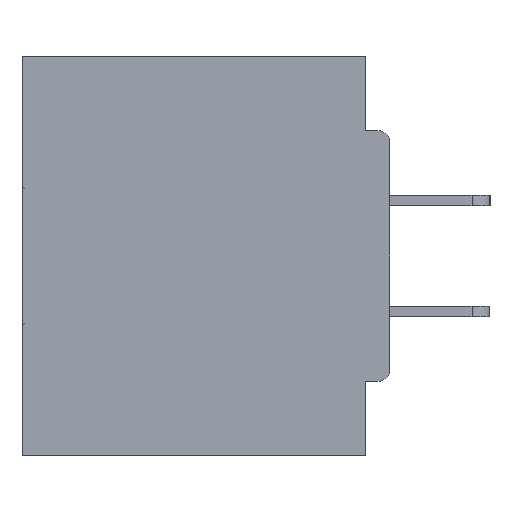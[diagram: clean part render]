
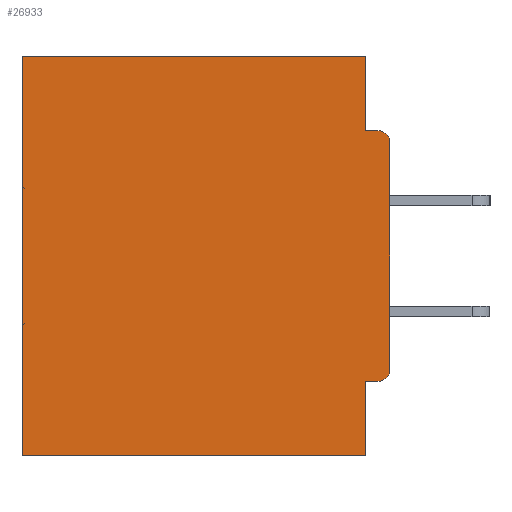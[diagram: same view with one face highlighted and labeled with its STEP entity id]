
A CAD part, left-side view. The second image highlights one B-rep face of the part: STEP entity #26933.
In plain terms, the highlighted planar face has unit normal (-1, 0, 0).
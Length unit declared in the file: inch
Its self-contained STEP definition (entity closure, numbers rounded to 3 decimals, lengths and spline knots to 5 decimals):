
#36 = FACE_OUTER_BOUND ( 'NONE', #34327, .T. ) ;
#632 = VERTEX_POINT ( 'NONE', #25162 ) ;
#668 = ORIENTED_EDGE ( 'NONE', *, *, #20912, .F. ) ;
#851 = ORIENTED_EDGE ( 'NONE', *, *, #15836, .T. ) ;
#2122 = DIRECTION ( 'NONE',  ( 0., 0., -1. ) ) ;
#2670 = LINE ( 'NONE', #19933, #12013 ) ;
#3550 = EDGE_CURVE ( 'NONE', #24531, #37569, #21996, .T. ) ;
#3868 = VERTEX_POINT ( 'NONE', #36581 ) ;
#4041 = CARTESIAN_POINT ( 'NONE',  ( 0.298, 0., 0. ) ) ;
#4188 = ORIENTED_EDGE ( 'NONE', *, *, #13792, .F. ) ;
#4927 = VERTEX_POINT ( 'NONE', #39853 ) ;
#5323 = AXIS2_PLACEMENT_3D ( 'NONE', #31454, #15018, #11538 ) ;
#5377 = CARTESIAN_POINT ( 'NONE',  ( 0.298, 0.015, -0.0935 ) ) ;
#5729 = CIRCLE ( 'NONE', #24705, 0.015 ) ;
#6074 = CARTESIAN_POINT ( 'NONE',  ( 0.298, 0., -0.1085 ) ) ;
#8146 = CARTESIAN_POINT ( 'NONE',  ( 0.298, 0., -0.0935 ) ) ;
#9762 = EDGE_CURVE ( 'NONE', #40306, #33398, #24197, .T. ) ;
#9853 = CARTESIAN_POINT ( 'NONE',  ( 0.298, 0.015, -0.3915 ) ) ;
#10743 = ORIENTED_EDGE ( 'NONE', *, *, #31924, .F. ) ;
#11538 = DIRECTION ( 'NONE',  ( 0., 0., -1. ) ) ;
#11604 = LINE ( 'NONE', #4041, #32440 ) ;
#11666 = ORIENTED_EDGE ( 'NONE', *, *, #3550, .T. ) ;
#11717 = VECTOR ( 'NONE', #26733, 39.37008 ) ;
#12013 = VECTOR ( 'NONE', #13821, 39.37008 ) ;
#12445 = EDGE_CURVE ( 'NONE', #35291, #37569, #16435, .T. ) ;
#12522 = ORIENTED_EDGE ( 'NONE', *, *, #34476, .F. ) ;
#13626 = VECTOR ( 'NONE', #2122, 39.37008 ) ;
#13642 = DIRECTION ( 'NONE',  ( -1., 0., 0. ) ) ;
#13781 = CARTESIAN_POINT ( 'NONE',  ( 0.298, 0.031, -0.5 ) ) ;
#13792 = EDGE_CURVE ( 'NONE', #20800, #33398, #34441, .T. ) ;
#13821 = DIRECTION ( 'NONE',  ( 0., 0., -1. ) ) ;
#15018 = DIRECTION ( 'NONE',  ( -1., 0., 0. ) ) ;
#15099 = DIRECTION ( 'NONE',  ( 0., 0., -1. ) ) ;
#15836 = EDGE_CURVE ( 'NONE', #632, #24531, #33780, .T. ) ;
#16435 = LINE ( 'NONE', #40356, #29423 ) ;
#17594 = DIRECTION ( 'NONE',  ( 1., 0., 0. ) ) ;
#19498 = LINE ( 'NONE', #13781, #11717 ) ;
#19933 = CARTESIAN_POINT ( 'NONE',  ( 0.298, 0.031, -0.5 ) ) ;
#20229 = CARTESIAN_POINT ( 'NONE',  ( 0.298, 0.031, -0.0935 ) ) ;
#20796 = DIRECTION ( 'NONE',  ( 0., 0., -1. ) ) ;
#20800 = VERTEX_POINT ( 'NONE', #20229 ) ;
#20912 = EDGE_CURVE ( 'NONE', #632, #20800, #2670, .T. ) ;
#21996 = LINE ( 'NONE', #34760, #13626 ) ;
#23482 = ORIENTED_EDGE ( 'NONE', *, *, #36048, .T. ) ;
#24197 = CIRCLE ( 'NONE', #5323, 0.015 ) ;
#24281 = CARTESIAN_POINT ( 'NONE',  ( 0.298, 0., 0. ) ) ;
#24529 = VECTOR ( 'NONE', #24626, 39.37008 ) ;
#24531 = VERTEX_POINT ( 'NONE', #30268 ) ;
#24626 = DIRECTION ( 'NONE',  ( 0., -1., 0. ) ) ;
#24705 = AXIS2_PLACEMENT_3D ( 'NONE', #9853, #13642, #36925 ) ;
#25162 = CARTESIAN_POINT ( 'NONE',  ( 0.298, 0.031, 0. ) ) ;
#26033 = DIRECTION ( 'NONE',  ( 0., 1., 0. ) ) ;
#26733 = DIRECTION ( 'NONE',  ( 0., 0., -1. ) ) ;
#26748 = CARTESIAN_POINT ( 'NONE',  ( 0.298, 0., -0.4065 ) ) ;
#26863 = CARTESIAN_POINT ( 'NONE',  ( 0.298, 0.031, -0.5 ) ) ;
#26933 = ADVANCED_FACE ( 'NONE', ( #36 ), #30552, .F. ) ;
#28036 = VECTOR ( 'NONE', #26033, 39.37008 ) ;
#28082 = AXIS2_PLACEMENT_3D ( 'NONE', #24281, #17594, #20796 ) ;
#28232 = ORIENTED_EDGE ( 'NONE', *, *, #33685, .F. ) ;
#29423 = VECTOR ( 'NONE', #40487, 39.37008 ) ;
#29830 = DIRECTION ( 'NONE',  ( 0., 1., 0. ) ) ;
#30268 = CARTESIAN_POINT ( 'NONE',  ( 0.298, 0.46, 0. ) ) ;
#30552 = PLANE ( 'NONE',  #28082 ) ;
#31454 = CARTESIAN_POINT ( 'NONE',  ( 0.298, 0.015, -0.1085 ) ) ;
#31924 = EDGE_CURVE ( 'NONE', #4927, #3868, #33124, .T. ) ;
#32440 = VECTOR ( 'NONE', #15099, 39.37008 ) ;
#32633 = VECTOR ( 'NONE', #29830, 39.37008 ) ;
#32708 = CARTESIAN_POINT ( 'NONE',  ( 0.298, 0., -0.3915 ) ) ;
#33124 = LINE ( 'NONE', #26748, #32633 ) ;
#33398 = VERTEX_POINT ( 'NONE', #5377 ) ;
#33685 = EDGE_CURVE ( 'NONE', #3868, #35291, #19498, .T. ) ;
#33760 = ORIENTED_EDGE ( 'NONE', *, *, #9762, .T. ) ;
#33780 = LINE ( 'NONE', #42642, #28036 ) ;
#34327 = EDGE_LOOP ( 'NONE', ( #33760, #4188, #668, #851, #11666, #34815, #28232, #10743, #23482, #12522 ) ) ;
#34441 = LINE ( 'NONE', #8146, #24529 ) ;
#34476 = EDGE_CURVE ( 'NONE', #40306, #40797, #11604, .T. ) ;
#34760 = CARTESIAN_POINT ( 'NONE',  ( 0.298, 0.46, 0. ) ) ;
#34815 = ORIENTED_EDGE ( 'NONE', *, *, #12445, .F. ) ;
#35291 = VERTEX_POINT ( 'NONE', #26863 ) ;
#36048 = EDGE_CURVE ( 'NONE', #4927, #40797, #5729, .T. ) ;
#36581 = CARTESIAN_POINT ( 'NONE',  ( 0.298, 0.031, -0.4065 ) ) ;
#36925 = DIRECTION ( 'NONE',  ( 0., 0., -1. ) ) ;
#37569 = VERTEX_POINT ( 'NONE', #42536 ) ;
#39853 = CARTESIAN_POINT ( 'NONE',  ( 0.298, 0.015, -0.4065 ) ) ;
#40306 = VERTEX_POINT ( 'NONE', #6074 ) ;
#40356 = CARTESIAN_POINT ( 'NONE',  ( 0.298, 0., -0.5 ) ) ;
#40487 = DIRECTION ( 'NONE',  ( 0., 1., 0. ) ) ;
#40797 = VERTEX_POINT ( 'NONE', #32708 ) ;
#42536 = CARTESIAN_POINT ( 'NONE',  ( 0.298, 0.46, -0.5 ) ) ;
#42642 = CARTESIAN_POINT ( 'NONE',  ( 0.298, 0., 0. ) ) ;
